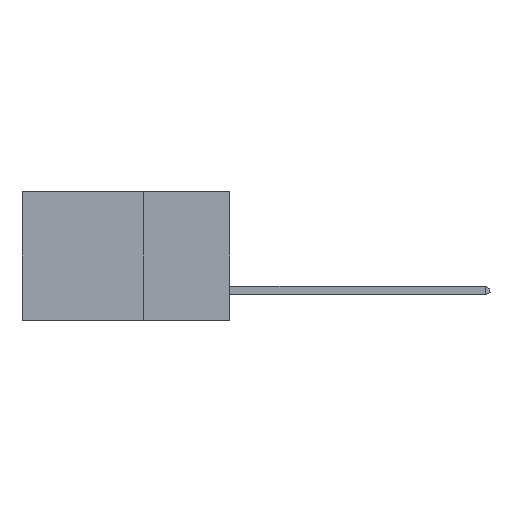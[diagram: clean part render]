
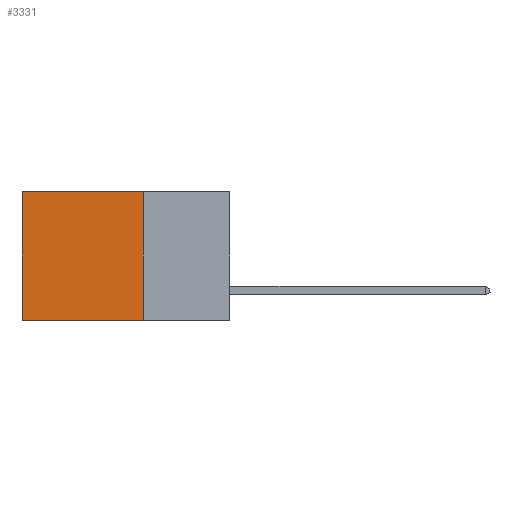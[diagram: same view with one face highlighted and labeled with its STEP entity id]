
A CAD part, left-side view. The second image highlights one B-rep face of the part: STEP entity #3331.
In plain terms, the highlighted planar face has unit normal (-1, 0, 0).
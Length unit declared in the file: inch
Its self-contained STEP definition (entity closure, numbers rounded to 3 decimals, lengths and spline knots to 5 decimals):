
#479 = CARTESIAN_POINT ( 'NONE',  ( 0.298, 0.25, -0.37 ) ) ;
#763 = LINE ( 'NONE', #11520, #6571 ) ;
#819 = EDGE_CURVE ( 'NONE', #3165, #7228, #2083, .T. ) ;
#845 = DIRECTION ( 'NONE',  ( 1., 0., 0. ) ) ;
#910 = LINE ( 'NONE', #8874, #11273 ) ;
#932 = VERTEX_POINT ( 'NONE', #1826 ) ;
#939 = CARTESIAN_POINT ( 'NONE',  ( 0.298, 0.6, 0. ) ) ;
#1283 = EDGE_CURVE ( 'NONE', #3165, #8322, #763, .T. ) ;
#1826 = CARTESIAN_POINT ( 'NONE',  ( 0.298, 0.6, -0.37 ) ) ;
#1866 = PLANE ( 'NONE',  #11592 ) ;
#2083 = LINE ( 'NONE', #10862, #10574 ) ;
#2647 = DIRECTION ( 'NONE',  ( 0., 0., -1. ) ) ;
#2678 = DIRECTION ( 'NONE',  ( 0., 1., 0. ) ) ;
#3165 = VERTEX_POINT ( 'NONE', #11215 ) ;
#3331 = ADVANCED_FACE ( 'NONE', ( #3664 ), #1866, .F. ) ;
#3664 = FACE_OUTER_BOUND ( 'NONE', #3756, .T. ) ;
#3756 = EDGE_LOOP ( 'NONE', ( #13504, #9951, #12556, #6731 ) ) ;
#4483 = DIRECTION ( 'NONE',  ( 0., 0., -1. ) ) ;
#4751 = LINE ( 'NONE', #479, #9739 ) ;
#6202 = DIRECTION ( 'NONE',  ( 0., 1., 0. ) ) ;
#6571 = VECTOR ( 'NONE', #6202, 39.37008 ) ;
#6731 = ORIENTED_EDGE ( 'NONE', *, *, #1283, .T. ) ;
#7228 = VERTEX_POINT ( 'NONE', #11990 ) ;
#7712 = DIRECTION ( 'NONE',  ( 0., 0., -1. ) ) ;
#7965 = CARTESIAN_POINT ( 'NONE',  ( 0.298, 0.25, 0. ) ) ;
#8322 = VERTEX_POINT ( 'NONE', #939 ) ;
#8874 = CARTESIAN_POINT ( 'NONE',  ( 0.298, 0.6, 0. ) ) ;
#9739 = VECTOR ( 'NONE', #2678, 39.37008 ) ;
#9951 = ORIENTED_EDGE ( 'NONE', *, *, #12252, .F. ) ;
#10574 = VECTOR ( 'NONE', #4483, 39.37008 ) ;
#10862 = CARTESIAN_POINT ( 'NONE',  ( 0.298, 0.25, 0. ) ) ;
#11215 = CARTESIAN_POINT ( 'NONE',  ( 0.298, 0.25, 0. ) ) ;
#11273 = VECTOR ( 'NONE', #7712, 39.37008 ) ;
#11520 = CARTESIAN_POINT ( 'NONE',  ( 0.298, 0.25, 0. ) ) ;
#11592 = AXIS2_PLACEMENT_3D ( 'NONE', #7965, #845, #2647 ) ;
#11764 = EDGE_CURVE ( 'NONE', #8322, #932, #910, .T. ) ;
#11990 = CARTESIAN_POINT ( 'NONE',  ( 0.298, 0.25, -0.37 ) ) ;
#12252 = EDGE_CURVE ( 'NONE', #7228, #932, #4751, .T. ) ;
#12556 = ORIENTED_EDGE ( 'NONE', *, *, #819, .F. ) ;
#13504 = ORIENTED_EDGE ( 'NONE', *, *, #11764, .T. ) ;
